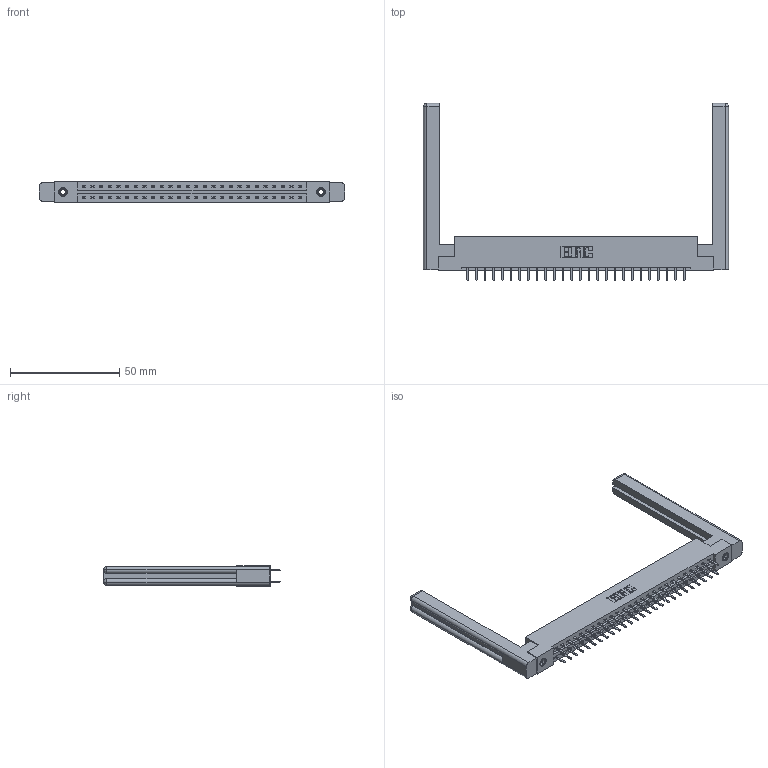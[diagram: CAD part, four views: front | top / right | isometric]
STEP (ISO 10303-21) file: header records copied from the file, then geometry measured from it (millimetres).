
FILE_DESCRIPTION (( 'STEP AP203' ), '1' );
FILE_NAME ('387-052-520-258.STEP', '2019-10-19T02:45:26', ( '' ), ( '' ), 'SwSTEP 2.0', 'SolidWorks 2016', '' );
FILE_SCHEMA (( 'CONFIG_CONTROL_DESIGN' ));
Length unit declared in the file: inch
Products named in the file (5): 307-220-058; 337 Part_Flush Mounting Lugs - 0.156 Dia-TI; 345-250-001_345-250-001-102; 387-052-520-258; 345-292-001_345-293-120
Assembly tree (57 placements, depth 2):
  387-052-520-258
    337 Part_Flush Mounting Lugs - 0.156 Dia-TI
    345-292-001_345-293-120  x52
    345-250-001_345-250-001-102  x2
    307-220-058  x2
Bounding box: 139.65 x 81.11 x 9.4 mm (x, y, z)
Volume: 21623.9 mm3; surface area: 21197.5 mm2
Topology: 57 solids, 57 shells, 3272 faces, 9453 edges, 6150 vertices
Faces by surface type: plane 2234, cylinder 1014, cone 12, torus 12
Entity records: 24976 total; most frequent: CARTESIAN_POINT 4241, ORIENTED_EDGE 4104, DIRECTION 3640, EDGE_CURVE 2052, LINE 1872, VECTOR 1872, VERTEX_POINT 1358, AXIS2_PLACEMENT_3D 884
